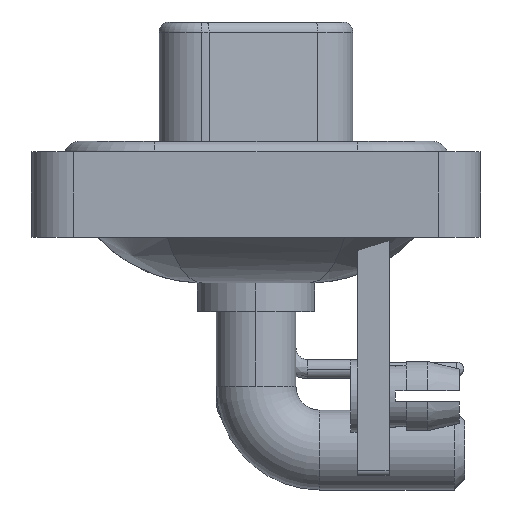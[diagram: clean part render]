
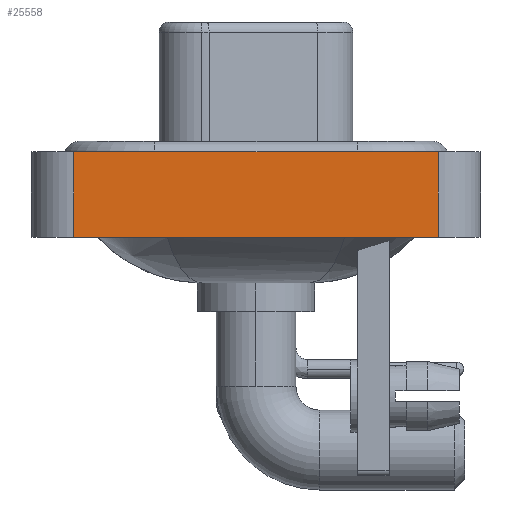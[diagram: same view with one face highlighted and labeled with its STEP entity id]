
A CAD part, left-side view. The second image highlights one B-rep face of the part: STEP entity #25558.
In plain terms, the highlighted planar face has unit normal (-1, 0, 0).
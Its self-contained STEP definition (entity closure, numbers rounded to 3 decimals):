
#23 = EDGE_CURVE ( 'NONE', #22601, #19760, #12369, .T. ) ;
#131 = CARTESIAN_POINT ( 'NONE',  ( -7.3, -8.55, -3.6 ) ) ;
#225 = EDGE_CURVE ( 'NONE', #22601, #18008, #26149, .T. ) ;
#1251 = CARTESIAN_POINT ( 'NONE',  ( -7.3, -8.55, 0.4 ) ) ;
#1352 = DIRECTION ( 'NONE',  ( 0., -1., 0. ) ) ;
#2782 = VECTOR ( 'NONE', #5454, 1000. ) ;
#2920 = AXIS2_PLACEMENT_3D ( 'NONE', #131, #10843, #8918 ) ;
#3765 = CARTESIAN_POINT ( 'NONE',  ( -7.3, -8.55, -3.6 ) ) ;
#4642 = VECTOR ( 'NONE', #12402, 1000. ) ;
#4841 = ORIENTED_EDGE ( 'NONE', *, *, #24534, .T. ) ;
#5454 = DIRECTION ( 'NONE',  ( 0., -1., 0. ) ) ;
#6410 = LINE ( 'NONE', #14737, #4642 ) ;
#6617 = PLANE ( 'NONE',  #2920 ) ;
#7186 = ORIENTED_EDGE ( 'NONE', *, *, #225, .T. ) ;
#7381 = CARTESIAN_POINT ( 'NONE',  ( -7.3, -8.55, 0.4 ) ) ;
#7873 = CARTESIAN_POINT ( 'NONE',  ( -7.3, 8.55, -3.6 ) ) ;
#8918 = DIRECTION ( 'NONE',  ( 0., 0., 1. ) ) ;
#9193 = EDGE_LOOP ( 'NONE', ( #4841, #10144, #23256, #7186 ) ) ;
#9460 = VECTOR ( 'NONE', #1352, 1000. ) ;
#10144 = ORIENTED_EDGE ( 'NONE', *, *, #17617, .F. ) ;
#10843 = DIRECTION ( 'NONE',  ( -1., 0., 0. ) ) ;
#11562 = LINE ( 'NONE', #1251, #2782 ) ;
#12369 = LINE ( 'NONE', #20876, #19397 ) ;
#12402 = DIRECTION ( 'NONE',  ( 0., 0., 1. ) ) ;
#12605 = FACE_OUTER_BOUND ( 'NONE', #9193, .T. ) ;
#13452 = CARTESIAN_POINT ( 'NONE',  ( -7.3, -8.55, -3.6 ) ) ;
#14737 = CARTESIAN_POINT ( 'NONE',  ( -7.3, -8.55, -3.6 ) ) ;
#17053 = VERTEX_POINT ( 'NONE', #7381 ) ;
#17617 = EDGE_CURVE ( 'NONE', #19760, #17053, #11562, .T. ) ;
#17941 = CARTESIAN_POINT ( 'NONE',  ( -7.3, 8.55, 0.4 ) ) ;
#18008 = VERTEX_POINT ( 'NONE', #3765 ) ;
#19397 = VECTOR ( 'NONE', #23045, 1000. ) ;
#19760 = VERTEX_POINT ( 'NONE', #17941 ) ;
#20876 = CARTESIAN_POINT ( 'NONE',  ( -7.3, 8.55, -3.6 ) ) ;
#22601 = VERTEX_POINT ( 'NONE', #7873 ) ;
#23045 = DIRECTION ( 'NONE',  ( 0., 0., 1. ) ) ;
#23256 = ORIENTED_EDGE ( 'NONE', *, *, #23, .F. ) ;
#24534 = EDGE_CURVE ( 'NONE', #18008, #17053, #6410, .T. ) ;
#25558 = ADVANCED_FACE ( 'NONE', ( #12605 ), #6617, .T. ) ;
#26149 = LINE ( 'NONE', #13452, #9460 ) ;
